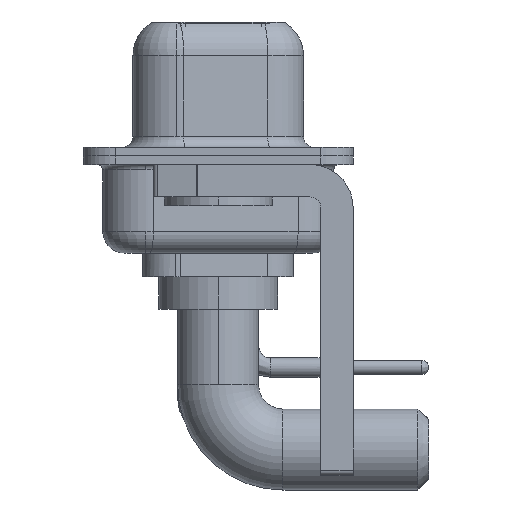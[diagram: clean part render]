
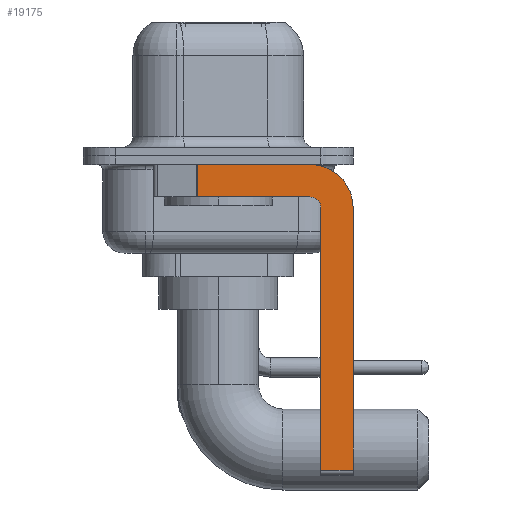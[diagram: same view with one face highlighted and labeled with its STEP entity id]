
A CAD part, left-side view. The second image highlights one B-rep face of the part: STEP entity #19175.
In plain terms, the highlighted planar face has unit normal (-1, 0, 0).
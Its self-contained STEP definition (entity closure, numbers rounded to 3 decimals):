
#478 = VECTOR ( 'NONE', #5530, 1000. ) ;
#486 = CARTESIAN_POINT ( 'NONE',  ( -2.9, -6.25, -2.4 ) ) ;
#1167 = FACE_OUTER_BOUND ( 'NONE', #11052, .T. ) ;
#1254 = LINE ( 'NONE', #14908, #6236 ) ;
#2478 = EDGE_CURVE ( 'NONE', #7645, #10313, #9057, .T. ) ;
#2674 = CARTESIAN_POINT ( 'NONE',  ( -2.9, -6.25, -14.55 ) ) ;
#2799 = CARTESIAN_POINT ( 'NONE',  ( -2.9, -4.25, -2.4 ) ) ;
#2827 = VECTOR ( 'NONE', #8350, 1000. ) ;
#3012 = DIRECTION ( 'NONE',  ( 0., 0., -1. ) ) ;
#3207 = VERTEX_POINT ( 'NONE', #486 ) ;
#3669 = AXIS2_PLACEMENT_3D ( 'NONE', #9540, #9329, #14011 ) ;
#4094 = ORIENTED_EDGE ( 'NONE', *, *, #4856, .F. ) ;
#4401 = VERTEX_POINT ( 'NONE', #12973 ) ;
#4536 = ORIENTED_EDGE ( 'NONE', *, *, #15310, .T. ) ;
#4856 = EDGE_CURVE ( 'NONE', #9977, #5473, #9877, .T. ) ;
#4950 = CARTESIAN_POINT ( 'NONE',  ( -2.9, -4.25, -1.9 ) ) ;
#5406 = ORIENTED_EDGE ( 'NONE', *, *, #2478, .F. ) ;
#5473 = VERTEX_POINT ( 'NONE', #13487 ) ;
#5530 = DIRECTION ( 'NONE',  ( 0., -1., 0. ) ) ;
#5608 = VERTEX_POINT ( 'NONE', #2674 ) ;
#6195 = DIRECTION ( 'NONE',  ( 1., 0., 0. ) ) ;
#6236 = VECTOR ( 'NONE', #3012, 1000. ) ;
#6294 = ORIENTED_EDGE ( 'NONE', *, *, #19622, .F. ) ;
#6613 = DIRECTION ( 'NONE',  ( 0., 0., 1. ) ) ;
#6925 = EDGE_CURVE ( 'NONE', #5473, #4401, #8143, .T. ) ;
#7301 = LINE ( 'NONE', #20509, #478 ) ;
#7645 = VERTEX_POINT ( 'NONE', #14290 ) ;
#8143 = LINE ( 'NONE', #4950, #2827 ) ;
#8350 = DIRECTION ( 'NONE',  ( 0., 1., 0. ) ) ;
#9057 = LINE ( 'NONE', #14075, #11130 ) ;
#9329 = DIRECTION ( 'NONE',  ( 1., 0., 0. ) ) ;
#9374 = DIRECTION ( 'NONE',  ( 0., 0., -1. ) ) ;
#9540 = CARTESIAN_POINT ( 'NONE',  ( -2.9, -4.25, -2.4 ) ) ;
#9877 = CIRCLE ( 'NONE', #18940, 0.5 ) ;
#9946 = EDGE_CURVE ( 'NONE', #10313, #3207, #13596, .T. ) ;
#9977 = VERTEX_POINT ( 'NONE', #12690 ) ;
#10037 = ORIENTED_EDGE ( 'NONE', *, *, #15263, .T. ) ;
#10255 = CARTESIAN_POINT ( 'NONE',  ( -2.9, -4.75, -14.55 ) ) ;
#10313 = VERTEX_POINT ( 'NONE', #20115 ) ;
#10984 = DIRECTION ( 'NONE',  ( 0., 0., 1. ) ) ;
#11052 = EDGE_LOOP ( 'NONE', ( #5406, #4536, #17382, #4094, #15453, #10037, #6294, #18446 ) ) ;
#11130 = VECTOR ( 'NONE', #12854, 1000. ) ;
#11317 = DIRECTION ( 'NONE',  ( -1., 0., 0. ) ) ;
#12596 = CARTESIAN_POINT ( 'NONE',  ( -2.9, -4.75, -14.8 ) ) ;
#12690 = CARTESIAN_POINT ( 'NONE',  ( -2.9, -4.75, -2.4 ) ) ;
#12854 = DIRECTION ( 'NONE',  ( 0., -1., 0. ) ) ;
#12973 = CARTESIAN_POINT ( 'NONE',  ( -2.9, 0.978, -1.9 ) ) ;
#13412 = VECTOR ( 'NONE', #9374, 1000. ) ;
#13487 = CARTESIAN_POINT ( 'NONE',  ( -2.9, -4.25, -1.9 ) ) ;
#13596 = CIRCLE ( 'NONE', #3669, 2. ) ;
#13921 = EDGE_CURVE ( 'NONE', #17544, #9977, #20822, .T. ) ;
#14011 = DIRECTION ( 'NONE',  ( 0., 0., -1. ) ) ;
#14075 = CARTESIAN_POINT ( 'NONE',  ( -2.9, 3., -0.4 ) ) ;
#14290 = CARTESIAN_POINT ( 'NONE',  ( -2.9, 0.978, -0.4 ) ) ;
#14908 = CARTESIAN_POINT ( 'NONE',  ( -2.9, -6.25, -2.4 ) ) ;
#15263 = EDGE_CURVE ( 'NONE', #17544, #5608, #7301, .T. ) ;
#15310 = EDGE_CURVE ( 'NONE', #7645, #4401, #19625, .T. ) ;
#15453 = ORIENTED_EDGE ( 'NONE', *, *, #13921, .F. ) ;
#16460 = PLANE ( 'NONE',  #21540 ) ;
#17190 = VECTOR ( 'NONE', #10984, 1000. ) ;
#17382 = ORIENTED_EDGE ( 'NONE', *, *, #6925, .F. ) ;
#17544 = VERTEX_POINT ( 'NONE', #10255 ) ;
#17765 = CARTESIAN_POINT ( 'NONE',  ( -2.9, 0.978, -1.9 ) ) ;
#18446 = ORIENTED_EDGE ( 'NONE', *, *, #9946, .F. ) ;
#18940 = AXIS2_PLACEMENT_3D ( 'NONE', #2799, #11317, #6613 ) ;
#19175 = ADVANCED_FACE ( 'NONE', ( #1167 ), #16460, .F. ) ;
#19622 = EDGE_CURVE ( 'NONE', #3207, #5608, #1254, .T. ) ;
#19625 = LINE ( 'NONE', #17765, #13412 ) ;
#19840 = DIRECTION ( 'NONE',  ( 0., 0., -1. ) ) ;
#20115 = CARTESIAN_POINT ( 'NONE',  ( -2.9, -4.25, -0.4 ) ) ;
#20509 = CARTESIAN_POINT ( 'NONE',  ( -2.9, -4.25, -14.55 ) ) ;
#20822 = LINE ( 'NONE', #12596, #17190 ) ;
#21170 = CARTESIAN_POINT ( 'NONE',  ( -2.9, -4.25, -2.4 ) ) ;
#21540 = AXIS2_PLACEMENT_3D ( 'NONE', #21170, #6195, #19840 ) ;
